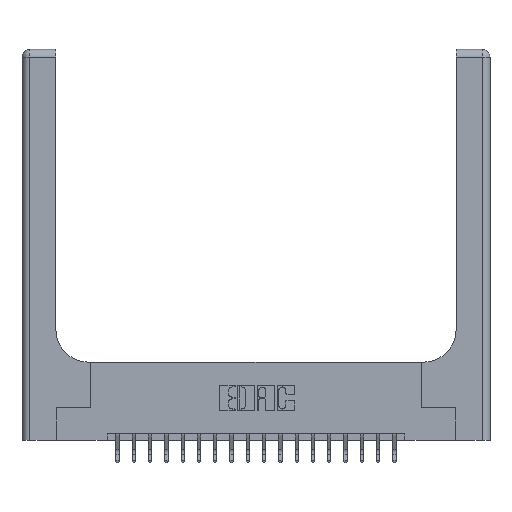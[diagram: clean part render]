
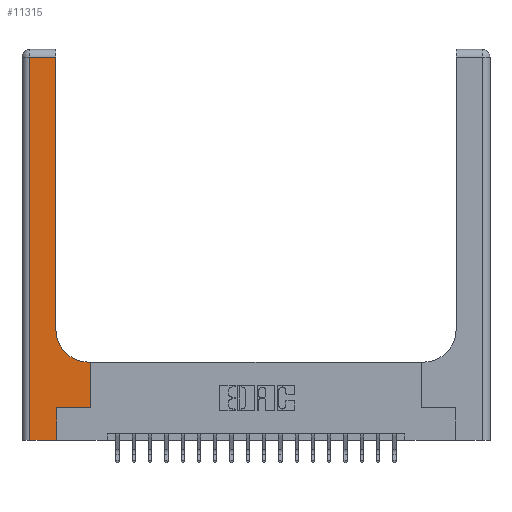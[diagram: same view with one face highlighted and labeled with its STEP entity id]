
A CAD part, top view. The second image highlights one B-rep face of the part: STEP entity #11315.
In plain terms, the highlighted planar face has unit normal (0, 0, 1).
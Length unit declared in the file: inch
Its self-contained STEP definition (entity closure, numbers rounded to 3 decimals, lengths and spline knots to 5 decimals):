
#102 = ORIENTED_EDGE ( 'NONE', *, *, #16649, .T. ) ;
#264 = LINE ( 'NONE', #5254, #19850 ) ;
#536 = DIRECTION ( 'NONE',  ( 1., 0., 0. ) ) ;
#554 = LINE ( 'NONE', #6811, #942 ) ;
#942 = VECTOR ( 'NONE', #8477, 39.37008 ) ;
#1002 = VERTEX_POINT ( 'NONE', #20314 ) ;
#1673 = EDGE_CURVE ( 'NONE', #9694, #1002, #9768, .T. ) ;
#1781 = VERTEX_POINT ( 'NONE', #5240 ) ;
#1927 = LINE ( 'NONE', #9569, #13848 ) ;
#2058 = EDGE_CURVE ( 'NONE', #17658, #8572, #554, .T. ) ;
#2187 = LINE ( 'NONE', #2303, #5046 ) ;
#2303 = CARTESIAN_POINT ( 'NONE',  ( 0.265, 0.25, 0.37 ) ) ;
#2663 = VERTEX_POINT ( 'NONE', #9575 ) ;
#2890 = ORIENTED_EDGE ( 'NONE', *, *, #11734, .T. ) ;
#3714 = EDGE_CURVE ( 'NONE', #1002, #1781, #2187, .T. ) ;
#3934 = EDGE_CURVE ( 'NONE', #20120, #17302, #264, .T. ) ;
#4086 = DIRECTION ( 'NONE',  ( 1., 0., 0. ) ) ;
#4818 = DIRECTION ( 'NONE',  ( 0., 1., 0. ) ) ;
#4830 = DIRECTION ( 'NONE',  ( 0., 0., -1. ) ) ;
#5046 = VECTOR ( 'NONE', #6961, 39.37008 ) ;
#5240 = CARTESIAN_POINT ( 'NONE',  ( 0.528, 0.25, 0.37 ) ) ;
#5254 = CARTESIAN_POINT ( 'NONE',  ( 0.26, 0.6, 0.37 ) ) ;
#5413 = ORIENTED_EDGE ( 'NONE', *, *, #3934, .T. ) ;
#5869 = DIRECTION ( 'NONE',  ( 0., 1., 0. ) ) ;
#6205 = ORIENTED_EDGE ( 'NONE', *, *, #20427, .T. ) ;
#6369 = ORIENTED_EDGE ( 'NONE', *, *, #3714, .T. ) ;
#6463 = CARTESIAN_POINT ( 'NONE',  ( 0.51, 0.6, 0.37 ) ) ;
#6793 = CARTESIAN_POINT ( 'NONE',  ( 0., 0., 0.37 ) ) ;
#6811 = CARTESIAN_POINT ( 'NONE',  ( 0.26, 3., 0.37 ) ) ;
#6961 = DIRECTION ( 'NONE',  ( 1., 0., 0. ) ) ;
#7476 = PLANE ( 'NONE',  #8526 ) ;
#7919 = VECTOR ( 'NONE', #5869, 39.37008 ) ;
#7920 = CARTESIAN_POINT ( 'NONE',  ( 0.26, 2.94, 0.37 ) ) ;
#8477 = DIRECTION ( 'NONE',  ( 0., 1., 0. ) ) ;
#8526 = AXIS2_PLACEMENT_3D ( 'NONE', #19277, #4830, #12645 ) ;
#8572 = VERTEX_POINT ( 'NONE', #7920 ) ;
#8589 = VERTEX_POINT ( 'NONE', #19185 ) ;
#8832 = CARTESIAN_POINT ( 'NONE',  ( 0.51, 0.85, 0.37 ) ) ;
#9263 = ORIENTED_EDGE ( 'NONE', *, *, #1673, .T. ) ;
#9371 = ORIENTED_EDGE ( 'NONE', *, *, #2058, .T. ) ;
#9569 = CARTESIAN_POINT ( 'NONE',  ( 0., 2.94, 0.37 ) ) ;
#9575 = CARTESIAN_POINT ( 'NONE',  ( 0.06, 0., 0.37 ) ) ;
#9694 = VERTEX_POINT ( 'NONE', #10729 ) ;
#9768 = LINE ( 'NONE', #12832, #12074 ) ;
#9857 = LINE ( 'NONE', #15828, #7919 ) ;
#9910 = DIRECTION ( 'NONE',  ( -1., 0., 0. ) ) ;
#9965 = CIRCLE ( 'NONE', #14369, 0.25 ) ;
#10030 = CARTESIAN_POINT ( 'NONE',  ( 0.528, 0.6, 0.37 ) ) ;
#10729 = CARTESIAN_POINT ( 'NONE',  ( 0.265, 0., 0.37 ) ) ;
#10881 = EDGE_LOOP ( 'NONE', ( #9371, #16686, #6205, #17920, #9263, #6369, #2890, #5413, #102 ) ) ;
#11315 = ADVANCED_FACE ( 'NONE', ( #15514 ), #7476, .F. ) ;
#11734 = EDGE_CURVE ( 'NONE', #1781, #20120, #9857, .T. ) ;
#12074 = VECTOR ( 'NONE', #4818, 39.37008 ) ;
#12443 = DIRECTION ( 'NONE',  ( 0., -1., 0. ) ) ;
#12645 = DIRECTION ( 'NONE',  ( -1., 0., 0. ) ) ;
#12832 = CARTESIAN_POINT ( 'NONE',  ( 0.265, 0., 0.37 ) ) ;
#12894 = EDGE_CURVE ( 'NONE', #2663, #9694, #14843, .T. ) ;
#13848 = VECTOR ( 'NONE', #19260, 39.37008 ) ;
#14255 = LINE ( 'NONE', #17513, #16917 ) ;
#14369 = AXIS2_PLACEMENT_3D ( 'NONE', #8832, #20079, #4086 ) ;
#14843 = LINE ( 'NONE', #6793, #16530 ) ;
#15514 = FACE_OUTER_BOUND ( 'NONE', #10881, .T. ) ;
#15828 = CARTESIAN_POINT ( 'NONE',  ( 0.528, 0.25, 0.37 ) ) ;
#16530 = VECTOR ( 'NONE', #536, 39.37008 ) ;
#16649 = EDGE_CURVE ( 'NONE', #17302, #17658, #9965, .T. ) ;
#16686 = ORIENTED_EDGE ( 'NONE', *, *, #19652, .T. ) ;
#16917 = VECTOR ( 'NONE', #12443, 39.37008 ) ;
#17302 = VERTEX_POINT ( 'NONE', #6463 ) ;
#17513 = CARTESIAN_POINT ( 'NONE',  ( 0.06, 3., 0.37 ) ) ;
#17658 = VERTEX_POINT ( 'NONE', #18906 ) ;
#17920 = ORIENTED_EDGE ( 'NONE', *, *, #12894, .T. ) ;
#18906 = CARTESIAN_POINT ( 'NONE',  ( 0.26, 0.85, 0.37 ) ) ;
#19185 = CARTESIAN_POINT ( 'NONE',  ( 0.06, 2.94, 0.37 ) ) ;
#19260 = DIRECTION ( 'NONE',  ( -1., 0., 0. ) ) ;
#19277 = CARTESIAN_POINT ( 'NONE',  ( 0., 3., 0.37 ) ) ;
#19652 = EDGE_CURVE ( 'NONE', #8572, #8589, #1927, .T. ) ;
#19850 = VECTOR ( 'NONE', #9910, 39.37008 ) ;
#20079 = DIRECTION ( 'NONE',  ( 0., 0., -1. ) ) ;
#20120 = VERTEX_POINT ( 'NONE', #10030 ) ;
#20314 = CARTESIAN_POINT ( 'NONE',  ( 0.265, 0.25, 0.37 ) ) ;
#20427 = EDGE_CURVE ( 'NONE', #8589, #2663, #14255, .T. ) ;
